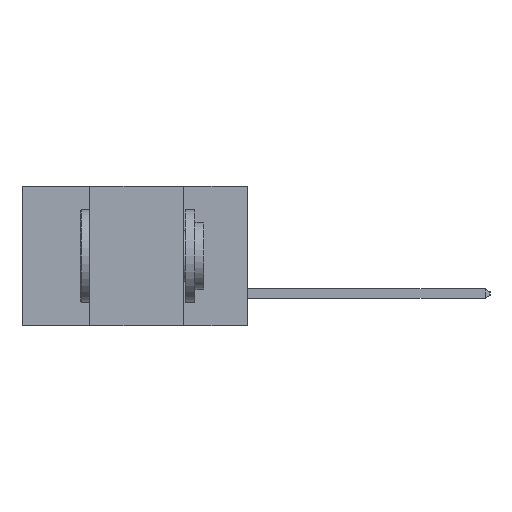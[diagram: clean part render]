
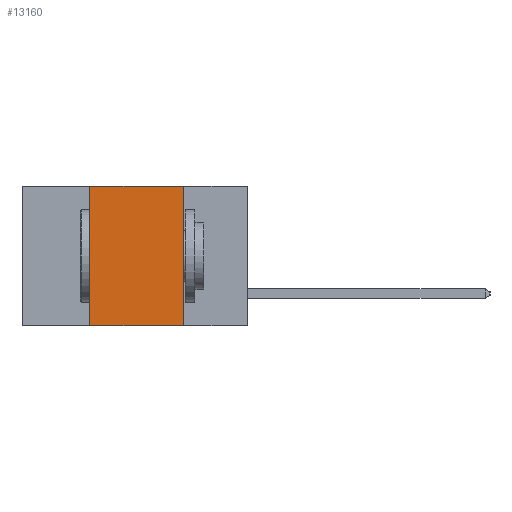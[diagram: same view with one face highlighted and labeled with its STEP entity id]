
A CAD part, left-side view. The second image highlights one B-rep face of the part: STEP entity #13160.
In plain terms, the highlighted planar face has unit normal (-1, 0, 0).
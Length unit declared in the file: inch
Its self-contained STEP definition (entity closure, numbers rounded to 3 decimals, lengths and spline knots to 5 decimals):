
#863 = CARTESIAN_POINT ( 'NONE',  ( 0., 0.17, -0.37 ) ) ;
#1245 = VECTOR ( 'NONE', #1990, 39.37008 ) ;
#1990 = DIRECTION ( 'NONE',  ( 0., -1., 0. ) ) ;
#2178 = CARTESIAN_POINT ( 'NONE',  ( 0., 0.6, -0.37 ) ) ;
#2290 = DIRECTION ( 'NONE',  ( 0., -1., 0. ) ) ;
#3033 = PLANE ( 'NONE',  #7514 ) ;
#3261 = CARTESIAN_POINT ( 'NONE',  ( 0., 0.17, 0. ) ) ;
#4491 = DIRECTION ( 'NONE',  ( 1., 0., 0. ) ) ;
#4927 = LINE ( 'NONE', #2178, #11413 ) ;
#5361 = FACE_OUTER_BOUND ( 'NONE', #9255, .T. ) ;
#5750 = LINE ( 'NONE', #5783, #9585 ) ;
#5783 = CARTESIAN_POINT ( 'NONE',  ( 0., 0.42, -0.37 ) ) ;
#5933 = VECTOR ( 'NONE', #10369, 39.37008 ) ;
#7514 = AXIS2_PLACEMENT_3D ( 'NONE', #12320, #4491, #13644 ) ;
#8307 = EDGE_CURVE ( 'NONE', #8607, #14991, #4927, .T. ) ;
#8607 = VERTEX_POINT ( 'NONE', #11239 ) ;
#9119 = EDGE_CURVE ( 'NONE', #8607, #13897, #5750, .T. ) ;
#9255 = EDGE_LOOP ( 'NONE', ( #13179, #16006, #15663, #15515 ) ) ;
#9585 = VECTOR ( 'NONE', #10880, 39.37008 ) ;
#9972 = EDGE_CURVE ( 'NONE', #13897, #13869, #15467, .T. ) ;
#10369 = DIRECTION ( 'NONE',  ( 0., 0., -1. ) ) ;
#10834 = EDGE_CURVE ( 'NONE', #13869, #14991, #12773, .T. ) ;
#10880 = DIRECTION ( 'NONE',  ( 0., 0., 1. ) ) ;
#11239 = CARTESIAN_POINT ( 'NONE',  ( 0., 0.42, -0.37 ) ) ;
#11362 = CARTESIAN_POINT ( 'NONE',  ( 0., 0.6, 0. ) ) ;
#11413 = VECTOR ( 'NONE', #2290, 39.37008 ) ;
#12320 = CARTESIAN_POINT ( 'NONE',  ( 0., 0.6, 0. ) ) ;
#12522 = CARTESIAN_POINT ( 'NONE',  ( 0., 0.42, 0. ) ) ;
#12773 = LINE ( 'NONE', #863, #5933 ) ;
#13160 = ADVANCED_FACE ( 'NONE', ( #5361 ), #3033, .F. ) ;
#13179 = ORIENTED_EDGE ( 'NONE', *, *, #10834, .F. ) ;
#13590 = CARTESIAN_POINT ( 'NONE',  ( 0., 0.17, -0.37 ) ) ;
#13644 = DIRECTION ( 'NONE',  ( 0., 0., -1. ) ) ;
#13869 = VERTEX_POINT ( 'NONE', #3261 ) ;
#13897 = VERTEX_POINT ( 'NONE', #12522 ) ;
#14991 = VERTEX_POINT ( 'NONE', #13590 ) ;
#15467 = LINE ( 'NONE', #11362, #1245 ) ;
#15515 = ORIENTED_EDGE ( 'NONE', *, *, #8307, .T. ) ;
#15663 = ORIENTED_EDGE ( 'NONE', *, *, #9119, .F. ) ;
#16006 = ORIENTED_EDGE ( 'NONE', *, *, #9972, .F. ) ;
